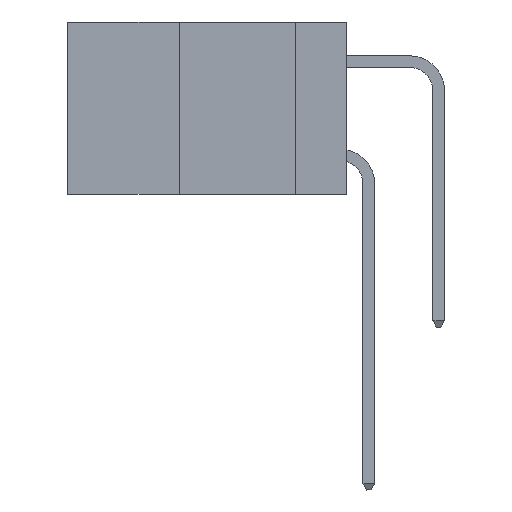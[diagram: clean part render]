
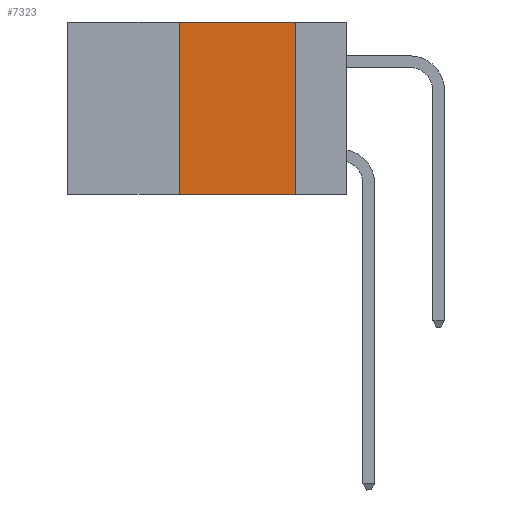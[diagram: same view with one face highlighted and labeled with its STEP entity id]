
A CAD part, left-side view. The second image highlights one B-rep face of the part: STEP entity #7323.
In plain terms, the highlighted planar face has unit normal (-1, 0, 0).
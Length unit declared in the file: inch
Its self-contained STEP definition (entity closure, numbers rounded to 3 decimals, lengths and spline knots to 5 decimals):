
#21 = VECTOR ( 'NONE', #5308, 39.37008 ) ;
#1888 = DIRECTION ( 'NONE',  ( 1., 0., 0. ) ) ;
#1980 = DIRECTION ( 'NONE',  ( 0., 0., 1. ) ) ;
#2094 = ORIENTED_EDGE ( 'NONE', *, *, #12017, .F. ) ;
#3968 = EDGE_LOOP ( 'NONE', ( #10577, #11392, #2094, #12226 ) ) ;
#4750 = LINE ( 'NONE', #10511, #21 ) ;
#5308 = DIRECTION ( 'NONE',  ( 0., -1., 0. ) ) ;
#5390 = LINE ( 'NONE', #15852, #14045 ) ;
#5589 = FACE_OUTER_BOUND ( 'NONE', #3968, .T. ) ;
#7323 = ADVANCED_FACE ( 'NONE', ( #5589 ), #12368, .F. ) ;
#7500 = CARTESIAN_POINT ( 'NONE',  ( 0., 0.6, -0.37 ) ) ;
#8185 = LINE ( 'NONE', #7500, #21728 ) ;
#8244 = VERTEX_POINT ( 'NONE', #14679 ) ;
#8939 = DIRECTION ( 'NONE',  ( 0., 0., -1. ) ) ;
#9852 = VERTEX_POINT ( 'NONE', #19140 ) ;
#10511 = CARTESIAN_POINT ( 'NONE',  ( 0., 0.6, 0. ) ) ;
#10577 = ORIENTED_EDGE ( 'NONE', *, *, #17699, .F. ) ;
#10642 = CARTESIAN_POINT ( 'NONE',  ( 0., 0.6, 0. ) ) ;
#10867 = EDGE_CURVE ( 'NONE', #9852, #17732, #8185, .T. ) ;
#10972 = VERTEX_POINT ( 'NONE', #12862 ) ;
#11392 = ORIENTED_EDGE ( 'NONE', *, *, #18279, .F. ) ;
#12017 = EDGE_CURVE ( 'NONE', #9852, #8244, #5390, .T. ) ;
#12129 = LINE ( 'NONE', #14106, #17175 ) ;
#12226 = ORIENTED_EDGE ( 'NONE', *, *, #10867, .T. ) ;
#12368 = PLANE ( 'NONE',  #16758 ) ;
#12862 = CARTESIAN_POINT ( 'NONE',  ( 0., 0.11, 0. ) ) ;
#14045 = VECTOR ( 'NONE', #1980, 39.37008 ) ;
#14065 = DIRECTION ( 'NONE',  ( 0., 0., -1. ) ) ;
#14106 = CARTESIAN_POINT ( 'NONE',  ( 0., 0.11, 0. ) ) ;
#14679 = CARTESIAN_POINT ( 'NONE',  ( 0., 0.36, 0. ) ) ;
#15852 = CARTESIAN_POINT ( 'NONE',  ( 0., 0.36, 0. ) ) ;
#16758 = AXIS2_PLACEMENT_3D ( 'NONE', #10642, #1888, #14065 ) ;
#17175 = VECTOR ( 'NONE', #8939, 39.37008 ) ;
#17592 = CARTESIAN_POINT ( 'NONE',  ( 0., 0.11, -0.37 ) ) ;
#17699 = EDGE_CURVE ( 'NONE', #10972, #17732, #12129, .T. ) ;
#17732 = VERTEX_POINT ( 'NONE', #17592 ) ;
#17747 = DIRECTION ( 'NONE',  ( 0., -1., 0. ) ) ;
#18279 = EDGE_CURVE ( 'NONE', #8244, #10972, #4750, .T. ) ;
#19140 = CARTESIAN_POINT ( 'NONE',  ( 0., 0.36, -0.37 ) ) ;
#21728 = VECTOR ( 'NONE', #17747, 39.37008 ) ;
